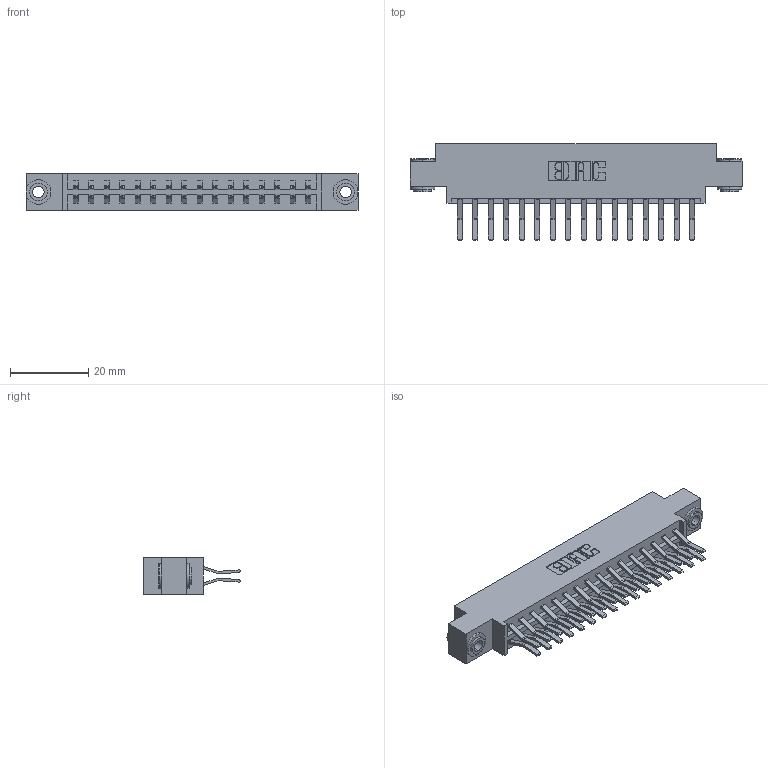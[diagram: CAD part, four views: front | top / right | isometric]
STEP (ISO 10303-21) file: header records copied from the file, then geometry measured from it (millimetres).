
FILE_DESCRIPTION (( 'STEP AP203' ), '1' );
FILE_NAME ('833-032-560-803.STEP', '2020-06-02T19:34:54', ( '' ), ( '' ), 'SwSTEP 2.0', 'SolidWorks 2020', '' );
FILE_SCHEMA (( 'CONFIG_CONTROL_DESIGN' ));
Length unit declared in the file: inch
Products named in the file (4): 833-032-560-803; 833 Part_Offset - .156 Dia - TH; 345-292-001_560 Tail; 345-250-002_345-250-002-102
Assembly tree (35 placements, depth 2):
  833-032-560-803
    833 Part_Offset - .156 Dia - TH
    345-292-001_560 Tail  x32
    345-250-002_345-250-002-102  x2
Bounding box: 84.94 x 24.78 x 9.4 mm (x, y, z)
Volume: 8429.8 mm3; surface area: 10726.8 mm2
Topology: 35 solids, 35 shells, 1884 faces, 5551 edges, 3654 vertices
Faces by surface type: plane 1236, cylinder 640, cone 8
Entity records: 14526 total; most frequent: CARTESIAN_POINT 2417, ORIENTED_EDGE 2346, DIRECTION 2147, EDGE_CURVE 1173, VECTOR 1017, LINE 1017, VERTEX_POINT 778, AXIS2_PLACEMENT_3D 565
